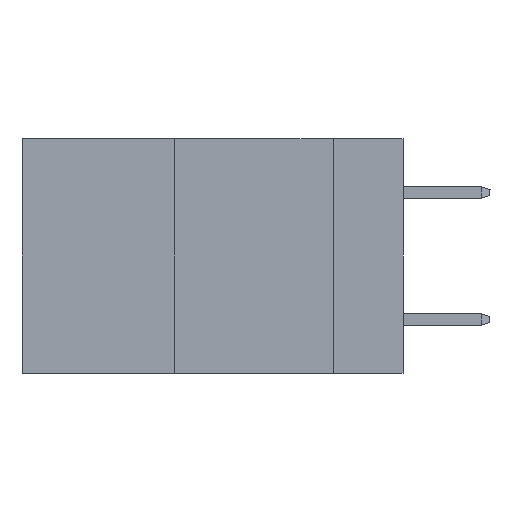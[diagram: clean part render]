
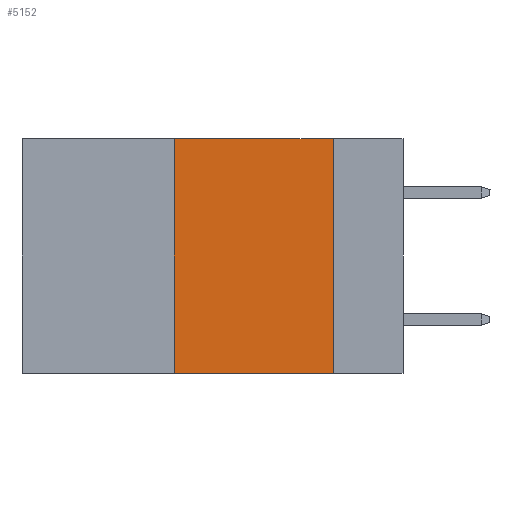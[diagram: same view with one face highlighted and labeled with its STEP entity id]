
A CAD part, left-side view. The second image highlights one B-rep face of the part: STEP entity #5152.
In plain terms, the highlighted planar face has unit normal (-1, 0, 0).
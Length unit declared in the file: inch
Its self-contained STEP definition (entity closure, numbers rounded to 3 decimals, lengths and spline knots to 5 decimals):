
#32 = DIRECTION ( 'NONE',  ( 0., -1., 0. ) ) ;
#65 = ORIENTED_EDGE ( 'NONE', *, *, #572, .F. ) ;
#161 = VECTOR ( 'NONE', #3236, 39.37008 ) ;
#326 = CARTESIAN_POINT ( 'NONE',  ( 0., 0.11, 0. ) ) ;
#572 = EDGE_CURVE ( 'NONE', #11230, #9018, #9545, .T. ) ;
#851 = LINE ( 'NONE', #10964, #1548 ) ;
#1301 = AXIS2_PLACEMENT_3D ( 'NONE', #6236, #8941, #11423 ) ;
#1548 = VECTOR ( 'NONE', #32, 39.37008 ) ;
#1790 = EDGE_LOOP ( 'NONE', ( #2910, #4522, #65, #7088 ) ) ;
#2910 = ORIENTED_EDGE ( 'NONE', *, *, #7630, .F. ) ;
#3126 = LINE ( 'NONE', #326, #11028 ) ;
#3236 = DIRECTION ( 'NONE',  ( 0., -1., 0. ) ) ;
#3569 = CARTESIAN_POINT ( 'NONE',  ( 0., 0.36, 0. ) ) ;
#3682 = EDGE_CURVE ( 'NONE', #11230, #7183, #10362, .T. ) ;
#3976 = DIRECTION ( 'NONE',  ( 0., 0., -1. ) ) ;
#4032 = CARTESIAN_POINT ( 'NONE',  ( 0., 0.36, 0. ) ) ;
#4472 = CARTESIAN_POINT ( 'NONE',  ( 0., 0.36, -0.37 ) ) ;
#4522 = ORIENTED_EDGE ( 'NONE', *, *, #6984, .F. ) ;
#5152 = ADVANCED_FACE ( 'NONE', ( #9770 ), #10538, .F. ) ;
#6236 = CARTESIAN_POINT ( 'NONE',  ( 0., 0.6, 0. ) ) ;
#6984 = EDGE_CURVE ( 'NONE', #9018, #9700, #851, .T. ) ;
#7088 = ORIENTED_EDGE ( 'NONE', *, *, #3682, .T. ) ;
#7183 = VERTEX_POINT ( 'NONE', #11545 ) ;
#7374 = VECTOR ( 'NONE', #11302, 39.37008 ) ;
#7630 = EDGE_CURVE ( 'NONE', #9700, #7183, #3126, .T. ) ;
#7792 = CARTESIAN_POINT ( 'NONE',  ( 0., 0.11, 0. ) ) ;
#8941 = DIRECTION ( 'NONE',  ( 1., 0., 0. ) ) ;
#9018 = VERTEX_POINT ( 'NONE', #3569 ) ;
#9537 = CARTESIAN_POINT ( 'NONE',  ( 0., 0.6, -0.37 ) ) ;
#9545 = LINE ( 'NONE', #4032, #7374 ) ;
#9700 = VERTEX_POINT ( 'NONE', #7792 ) ;
#9770 = FACE_OUTER_BOUND ( 'NONE', #1790, .T. ) ;
#10362 = LINE ( 'NONE', #9537, #161 ) ;
#10538 = PLANE ( 'NONE',  #1301 ) ;
#10964 = CARTESIAN_POINT ( 'NONE',  ( 0., 0.6, 0. ) ) ;
#11028 = VECTOR ( 'NONE', #3976, 39.37008 ) ;
#11230 = VERTEX_POINT ( 'NONE', #4472 ) ;
#11302 = DIRECTION ( 'NONE',  ( 0., 0., 1. ) ) ;
#11423 = DIRECTION ( 'NONE',  ( 0., 0., -1. ) ) ;
#11545 = CARTESIAN_POINT ( 'NONE',  ( 0., 0.11, -0.37 ) ) ;
